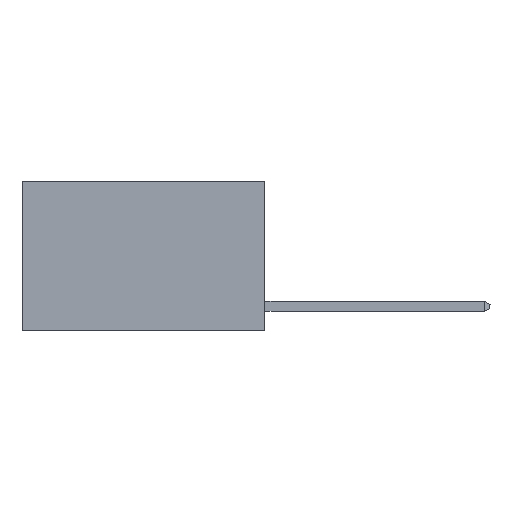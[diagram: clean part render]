
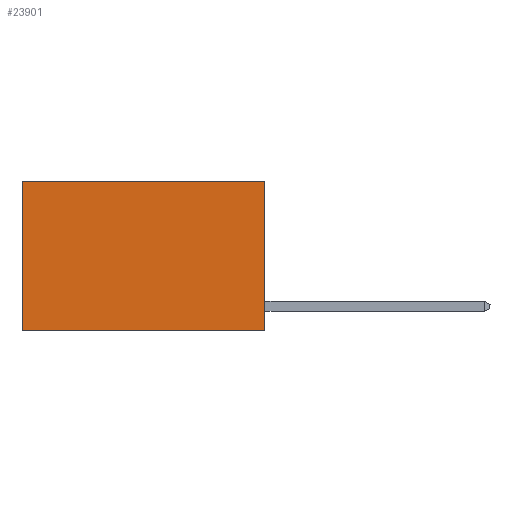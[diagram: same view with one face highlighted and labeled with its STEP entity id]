
A CAD part, left-side view. The second image highlights one B-rep face of the part: STEP entity #23901.
In plain terms, the highlighted planar face has unit normal (-1, 0, 0).
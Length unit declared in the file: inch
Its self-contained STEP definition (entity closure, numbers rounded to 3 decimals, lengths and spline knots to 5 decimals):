
#614 = EDGE_CURVE ( 'NONE', #20453, #16493, #18227, .T. ) ;
#702 = CARTESIAN_POINT ( 'NONE',  ( 0.2625, 0., 0. ) ) ;
#716 = CARTESIAN_POINT ( 'NONE',  ( 0.2625, 0., 0. ) ) ;
#1444 = EDGE_CURVE ( 'NONE', #20453, #6213, #5576, .T. ) ;
#2506 = ORIENTED_EDGE ( 'NONE', *, *, #9804, .T. ) ;
#3274 = ORIENTED_EDGE ( 'NONE', *, *, #1444, .T. ) ;
#4230 = DIRECTION ( 'NONE',  ( 0., 0., -1. ) ) ;
#4555 = CARTESIAN_POINT ( 'NONE',  ( 0.2625, 0., 0. ) ) ;
#5448 = DIRECTION ( 'NONE',  ( 0., 1., 0. ) ) ;
#5576 = LINE ( 'NONE', #716, #21121 ) ;
#6181 = CARTESIAN_POINT ( 'NONE',  ( 0.2625, 0.6, 0. ) ) ;
#6213 = VERTEX_POINT ( 'NONE', #7858 ) ;
#6361 = PLANE ( 'NONE',  #15893 ) ;
#7858 = CARTESIAN_POINT ( 'NONE',  ( 0.2625, 0.6, 0. ) ) ;
#8395 = DIRECTION ( 'NONE',  ( 0., 0., -1. ) ) ;
#8689 = ORIENTED_EDGE ( 'NONE', *, *, #614, .F. ) ;
#9804 = EDGE_CURVE ( 'NONE', #6213, #10837, #13853, .T. ) ;
#9868 = EDGE_CURVE ( 'NONE', #16493, #10837, #21182, .T. ) ;
#10837 = VERTEX_POINT ( 'NONE', #19382 ) ;
#12398 = VECTOR ( 'NONE', #5448, 39.37008 ) ;
#12975 = VECTOR ( 'NONE', #16141, 39.37008 ) ;
#13853 = LINE ( 'NONE', #6181, #24122 ) ;
#14629 = ORIENTED_EDGE ( 'NONE', *, *, #9868, .F. ) ;
#15448 = DIRECTION ( 'NONE',  ( 1., 0., 0. ) ) ;
#15893 = AXIS2_PLACEMENT_3D ( 'NONE', #4555, #15448, #4230 ) ;
#16141 = DIRECTION ( 'NONE',  ( 0., 0., -1. ) ) ;
#16493 = VERTEX_POINT ( 'NONE', #22190 ) ;
#16640 = CARTESIAN_POINT ( 'NONE',  ( 0.2625, 0., -0.37 ) ) ;
#17942 = CARTESIAN_POINT ( 'NONE',  ( 0.2625, 0., 0. ) ) ;
#18227 = LINE ( 'NONE', #17942, #12975 ) ;
#19382 = CARTESIAN_POINT ( 'NONE',  ( 0.2625, 0.6, -0.37 ) ) ;
#20316 = EDGE_LOOP ( 'NONE', ( #2506, #14629, #8689, #3274 ) ) ;
#20453 = VERTEX_POINT ( 'NONE', #702 ) ;
#21121 = VECTOR ( 'NONE', #23283, 39.37008 ) ;
#21182 = LINE ( 'NONE', #16640, #12398 ) ;
#22190 = CARTESIAN_POINT ( 'NONE',  ( 0.2625, 0., -0.37 ) ) ;
#23283 = DIRECTION ( 'NONE',  ( 0., 1., 0. ) ) ;
#23388 = FACE_OUTER_BOUND ( 'NONE', #20316, .T. ) ;
#23901 = ADVANCED_FACE ( 'NONE', ( #23388 ), #6361, .F. ) ;
#24122 = VECTOR ( 'NONE', #8395, 39.37008 ) ;
